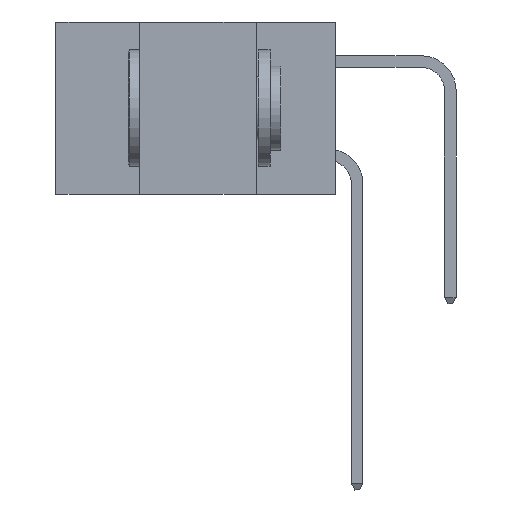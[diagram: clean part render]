
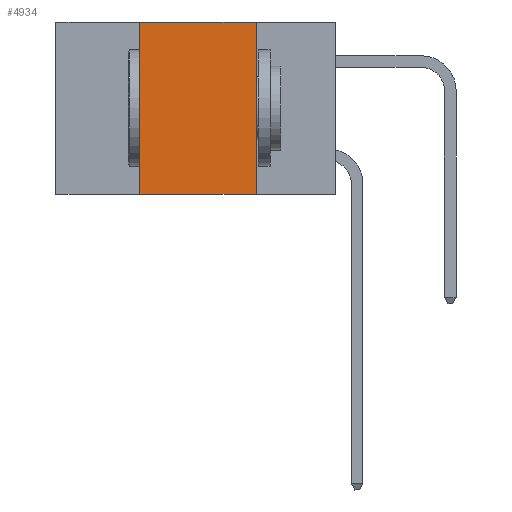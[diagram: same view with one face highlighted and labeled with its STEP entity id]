
A CAD part, left-side view. The second image highlights one B-rep face of the part: STEP entity #4934.
In plain terms, the highlighted planar face has unit normal (-1, 0, 0).
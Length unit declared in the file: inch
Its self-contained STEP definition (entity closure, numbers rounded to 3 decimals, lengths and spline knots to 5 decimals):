
#196 = LINE ( 'NONE', #2109, #11044 ) ;
#781 = ORIENTED_EDGE ( 'NONE', *, *, #10473, .F. ) ;
#1073 = CARTESIAN_POINT ( 'NONE',  ( 0., 0.17, -0.37 ) ) ;
#1271 = DIRECTION ( 'NONE',  ( 1., 0., 0. ) ) ;
#1419 = DIRECTION ( 'NONE',  ( 0., -1., 0. ) ) ;
#1630 = ORIENTED_EDGE ( 'NONE', *, *, #3792, .F. ) ;
#1780 = VECTOR ( 'NONE', #9381, 39.37008 ) ;
#2109 = CARTESIAN_POINT ( 'NONE',  ( 0., 0.6, 0. ) ) ;
#2499 = VECTOR ( 'NONE', #6486, 39.37008 ) ;
#2526 = CARTESIAN_POINT ( 'NONE',  ( 0., 0.42, 0. ) ) ;
#2566 = VERTEX_POINT ( 'NONE', #1073 ) ;
#2942 = DIRECTION ( 'NONE',  ( 0., -1., 0. ) ) ;
#3277 = VERTEX_POINT ( 'NONE', #7658 ) ;
#3439 = CARTESIAN_POINT ( 'NONE',  ( 0., 0.42, 0. ) ) ;
#3792 = EDGE_CURVE ( 'NONE', #3277, #2566, #10854, .T. ) ;
#4216 = EDGE_CURVE ( 'NONE', #5975, #2566, #4518, .T. ) ;
#4518 = LINE ( 'NONE', #9331, #10985 ) ;
#4934 = ADVANCED_FACE ( 'NONE', ( #8508 ), #10869, .F. ) ;
#5728 = CARTESIAN_POINT ( 'NONE',  ( 0., 0.6, 0. ) ) ;
#5975 = VERTEX_POINT ( 'NONE', #8921 ) ;
#6038 = AXIS2_PLACEMENT_3D ( 'NONE', #5728, #1271, #6565 ) ;
#6486 = DIRECTION ( 'NONE',  ( 0., 0., -1. ) ) ;
#6565 = DIRECTION ( 'NONE',  ( 0., 0., -1. ) ) ;
#6707 = VERTEX_POINT ( 'NONE', #3439 ) ;
#6958 = EDGE_LOOP ( 'NONE', ( #1630, #10006, #781, #11254 ) ) ;
#7000 = LINE ( 'NONE', #2526, #1780 ) ;
#7658 = CARTESIAN_POINT ( 'NONE',  ( 0., 0.17, 0. ) ) ;
#8398 = EDGE_CURVE ( 'NONE', #6707, #3277, #196, .T. ) ;
#8508 = FACE_OUTER_BOUND ( 'NONE', #6958, .T. ) ;
#8921 = CARTESIAN_POINT ( 'NONE',  ( 0., 0.42, -0.37 ) ) ;
#9331 = CARTESIAN_POINT ( 'NONE',  ( 0., 0.6, -0.37 ) ) ;
#9381 = DIRECTION ( 'NONE',  ( 0., 0., 1. ) ) ;
#10006 = ORIENTED_EDGE ( 'NONE', *, *, #8398, .F. ) ;
#10025 = CARTESIAN_POINT ( 'NONE',  ( 0., 0.17, 0. ) ) ;
#10473 = EDGE_CURVE ( 'NONE', #5975, #6707, #7000, .T. ) ;
#10854 = LINE ( 'NONE', #10025, #2499 ) ;
#10869 = PLANE ( 'NONE',  #6038 ) ;
#10985 = VECTOR ( 'NONE', #1419, 39.37008 ) ;
#11044 = VECTOR ( 'NONE', #2942, 39.37008 ) ;
#11254 = ORIENTED_EDGE ( 'NONE', *, *, #4216, .T. ) ;
